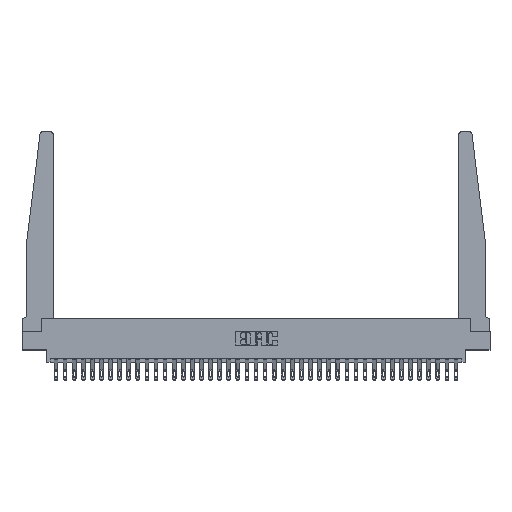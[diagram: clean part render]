
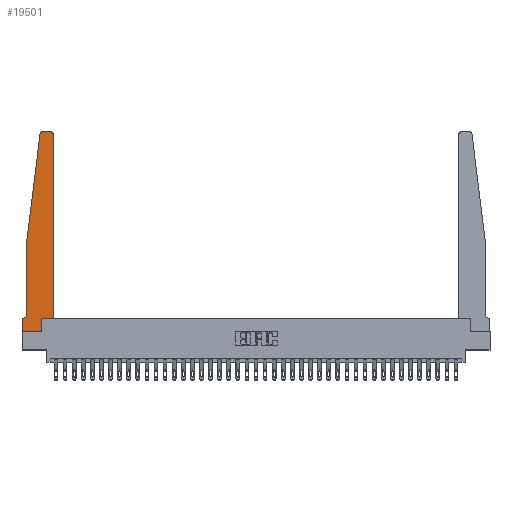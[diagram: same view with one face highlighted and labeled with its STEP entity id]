
A CAD part, top view. The second image highlights one B-rep face of the part: STEP entity #19501.
In plain terms, the highlighted planar face has unit normal (0, 0, 1).
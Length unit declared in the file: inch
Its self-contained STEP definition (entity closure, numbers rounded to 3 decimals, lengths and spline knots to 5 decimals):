
#413 = EDGE_LOOP ( 'NONE', ( #21265, #11486, #27851, #23254, #29439, #31000, #12179, #5132, #11664, #23606, #1675, #1129 ) ) ;
#449 = VERTEX_POINT ( 'NONE', #19975 ) ;
#647 = LINE ( 'NONE', #3462, #25666 ) ;
#704 = LINE ( 'NONE', #27752, #32612 ) ;
#1129 = ORIENTED_EDGE ( 'NONE', *, *, #28647, .T. ) ;
#1351 = CARTESIAN_POINT ( 'NONE',  ( 0.065, 0.1875, 0.37 ) ) ;
#1651 = CARTESIAN_POINT ( 'NONE',  ( 0.015, 0.2375, 0.37 ) ) ;
#1675 = ORIENTED_EDGE ( 'NONE', *, *, #21539, .T. ) ;
#2438 = CARTESIAN_POINT ( 'NONE',  ( 0., 0.1875, 0.37 ) ) ;
#2658 = CARTESIAN_POINT ( 'NONE',  ( 0.065, 0.2375, 0.37 ) ) ;
#2662 = VECTOR ( 'NONE', #22756, 39.37008 ) ;
#3230 = DIRECTION ( 'NONE',  ( 0., 0., 1. ) ) ;
#3462 = CARTESIAN_POINT ( 'NONE',  ( 0.2605, 0.18, 0.37 ) ) ;
#4801 = CARTESIAN_POINT ( 'NONE',  ( 0.395, 2.75, 0.37 ) ) ;
#4929 = VERTEX_POINT ( 'NONE', #26272 ) ;
#5116 = LINE ( 'NONE', #21244, #21145 ) ;
#5132 = ORIENTED_EDGE ( 'NONE', *, *, #29293, .T. ) ;
#5247 = PLANE ( 'NONE',  #15552 ) ;
#5414 = CARTESIAN_POINT ( 'NONE',  ( 0., 0., 0.37 ) ) ;
#5927 = VERTEX_POINT ( 'NONE', #2658 ) ;
#6226 = CARTESIAN_POINT ( 'NONE',  ( 0.425, 2.72, 0.37 ) ) ;
#6275 = CARTESIAN_POINT ( 'NONE',  ( 0.27653, 2.75, 0.37 ) ) ;
#6579 = DIRECTION ( 'NONE',  ( -1., 0., 0. ) ) ;
#6843 = CARTESIAN_POINT ( 'NONE',  ( 0.2605, 0., 0.37 ) ) ;
#7055 = CARTESIAN_POINT ( 'NONE',  ( 0.395, 2.72, 0.37 ) ) ;
#7393 = LINE ( 'NONE', #31428, #9317 ) ;
#8063 = VERTEX_POINT ( 'NONE', #19716 ) ;
#8744 = LINE ( 'NONE', #16616, #25414 ) ;
#8850 = CARTESIAN_POINT ( 'NONE',  ( 0.27653, 2.72, 0.37 ) ) ;
#9317 = VECTOR ( 'NONE', #18087, 39.37008 ) ;
#9657 = EDGE_CURVE ( 'NONE', #5927, #449, #21919, .T. ) ;
#9796 = LINE ( 'NONE', #1351, #2662 ) ;
#10407 = CARTESIAN_POINT ( 'NONE',  ( 0.065, 1.25, 0.37 ) ) ;
#10823 = DIRECTION ( 'NONE',  ( 0., 1., 0. ) ) ;
#10869 = FACE_OUTER_BOUND ( 'NONE', #413, .T. ) ;
#11486 = ORIENTED_EDGE ( 'NONE', *, *, #21250, .T. ) ;
#11664 = ORIENTED_EDGE ( 'NONE', *, *, #19651, .T. ) ;
#12179 = ORIENTED_EDGE ( 'NONE', *, *, #17488, .T. ) ;
#12240 = EDGE_CURVE ( 'NONE', #8063, #26905, #8744, .T. ) ;
#12311 = AXIS2_PLACEMENT_3D ( 'NONE', #8850, #3230, #13946 ) ;
#13162 = DIRECTION ( 'NONE',  ( 0., 0., 1. ) ) ;
#13946 = DIRECTION ( 'NONE',  ( 1., 0., 0. ) ) ;
#14169 = DIRECTION ( 'NONE',  ( 0., 1., 0. ) ) ;
#15466 = LINE ( 'NONE', #21428, #24425 ) ;
#15513 = EDGE_CURVE ( 'NONE', #18353, #17723, #15466, .T. ) ;
#15552 = AXIS2_PLACEMENT_3D ( 'NONE', #2438, #13162, #21199 ) ;
#16189 = CARTESIAN_POINT ( 'NONE',  ( 0., 0.1875, 0.37 ) ) ;
#16315 = DIRECTION ( 'NONE',  ( 0., -1., 0. ) ) ;
#16320 = VECTOR ( 'NONE', #29286, 39.37008 ) ;
#16616 = CARTESIAN_POINT ( 'NONE',  ( 0.425, 0.18, 0.37 ) ) ;
#16746 = VECTOR ( 'NONE', #10823, 39.37008 ) ;
#16840 = AXIS2_PLACEMENT_3D ( 'NONE', #7055, #25474, #23524 ) ;
#16852 = VERTEX_POINT ( 'NONE', #10407 ) ;
#17488 = EDGE_CURVE ( 'NONE', #19853, #4929, #7393, .T. ) ;
#17723 = VERTEX_POINT ( 'NONE', #6275 ) ;
#18087 = DIRECTION ( 'NONE',  ( 0., -1., 0. ) ) ;
#18301 = VERTEX_POINT ( 'NONE', #6226 ) ;
#18353 = VERTEX_POINT ( 'NONE', #4801 ) ;
#19011 = CIRCLE ( 'NONE', #12311, 0.03 ) ;
#19054 = EDGE_CURVE ( 'NONE', #16852, #5927, #5116, .T. ) ;
#19265 = DIRECTION ( 'NONE',  ( 1., 0., 0. ) ) ;
#19313 = DIRECTION ( 'NONE',  ( -0.122, -0.992, 0. ) ) ;
#19501 = ADVANCED_FACE ( 'NONE', ( #10869 ), #5247, .T. ) ;
#19651 = EDGE_CURVE ( 'NONE', #29174, #8063, #647, .T. ) ;
#19716 = CARTESIAN_POINT ( 'NONE',  ( 0.2605, 0.18, 0.37 ) ) ;
#19853 = VERTEX_POINT ( 'NONE', #16189 ) ;
#19975 = CARTESIAN_POINT ( 'NONE',  ( 0.015, 0.1875, 0.37 ) ) ;
#20433 = DIRECTION ( 'NONE',  ( 0., 0., -1. ) ) ;
#20589 = CARTESIAN_POINT ( 'NONE',  ( 0.425, 0.18, 0.37 ) ) ;
#21145 = VECTOR ( 'NONE', #16315, 39.37008 ) ;
#21199 = DIRECTION ( 'NONE',  ( 1., 0., 0. ) ) ;
#21244 = CARTESIAN_POINT ( 'NONE',  ( 0.065, 1.25, 0.37 ) ) ;
#21250 = EDGE_CURVE ( 'NONE', #17723, #31048, #19011, .T. ) ;
#21265 = ORIENTED_EDGE ( 'NONE', *, *, #15513, .T. ) ;
#21428 = CARTESIAN_POINT ( 'NONE',  ( 0.25, 2.75, 0.37 ) ) ;
#21539 = EDGE_CURVE ( 'NONE', #26905, #18301, #29921, .T. ) ;
#21919 = CIRCLE ( 'NONE', #26979, 0.05 ) ;
#22176 = CARTESIAN_POINT ( 'NONE',  ( 0.425, 0.18, 0.37 ) ) ;
#22549 = EDGE_CURVE ( 'NONE', #449, #19853, #9796, .T. ) ;
#22756 = DIRECTION ( 'NONE',  ( -1., 0., 0. ) ) ;
#23254 = ORIENTED_EDGE ( 'NONE', *, *, #19054, .T. ) ;
#23524 = DIRECTION ( 'NONE',  ( 1., 0., 0. ) ) ;
#23606 = ORIENTED_EDGE ( 'NONE', *, *, #12240, .T. ) ;
#24425 = VECTOR ( 'NONE', #26367, 39.37008 ) ;
#25414 = VECTOR ( 'NONE', #19265, 39.37008 ) ;
#25474 = DIRECTION ( 'NONE',  ( 0., 0., 1. ) ) ;
#25666 = VECTOR ( 'NONE', #14169, 39.37008 ) ;
#26272 = CARTESIAN_POINT ( 'NONE',  ( 0., 0., 0.37 ) ) ;
#26367 = DIRECTION ( 'NONE',  ( -1., 0., 0. ) ) ;
#26824 = LINE ( 'NONE', #5414, #16320 ) ;
#26905 = VERTEX_POINT ( 'NONE', #20589 ) ;
#26979 = AXIS2_PLACEMENT_3D ( 'NONE', #1651, #20433, #6579 ) ;
#27520 = CIRCLE ( 'NONE', #16840, 0.03 ) ;
#27752 = CARTESIAN_POINT ( 'NONE',  ( 0.065, 1.25, 0.37 ) ) ;
#27851 = ORIENTED_EDGE ( 'NONE', *, *, #30066, .T. ) ;
#28319 = CARTESIAN_POINT ( 'NONE',  ( 0.24675, 2.72367, 0.37 ) ) ;
#28647 = EDGE_CURVE ( 'NONE', #18301, #18353, #27520, .T. ) ;
#29174 = VERTEX_POINT ( 'NONE', #6843 ) ;
#29286 = DIRECTION ( 'NONE',  ( 1., 0., 0. ) ) ;
#29293 = EDGE_CURVE ( 'NONE', #4929, #29174, #26824, .T. ) ;
#29439 = ORIENTED_EDGE ( 'NONE', *, *, #9657, .T. ) ;
#29921 = LINE ( 'NONE', #22176, #16746 ) ;
#30066 = EDGE_CURVE ( 'NONE', #31048, #16852, #704, .T. ) ;
#31000 = ORIENTED_EDGE ( 'NONE', *, *, #22549, .T. ) ;
#31048 = VERTEX_POINT ( 'NONE', #28319 ) ;
#31428 = CARTESIAN_POINT ( 'NONE',  ( 0., 0., 0.37 ) ) ;
#32612 = VECTOR ( 'NONE', #19313, 39.37008 ) ;
